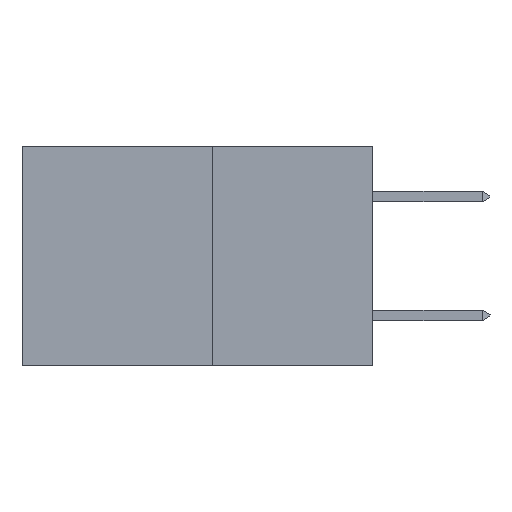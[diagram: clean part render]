
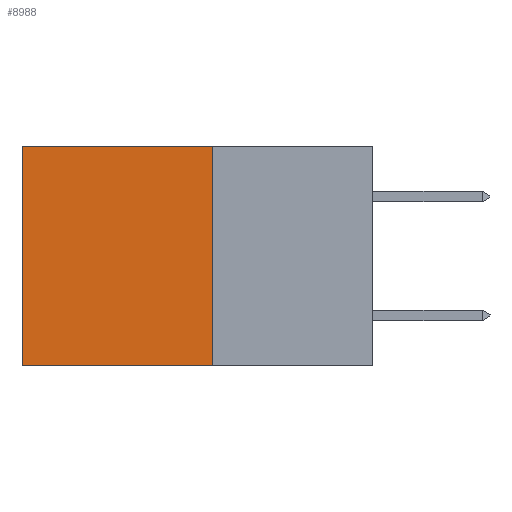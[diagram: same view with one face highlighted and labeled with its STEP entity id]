
A CAD part, left-side view. The second image highlights one B-rep face of the part: STEP entity #8988.
In plain terms, the highlighted planar face has unit normal (-1, 0, 0).
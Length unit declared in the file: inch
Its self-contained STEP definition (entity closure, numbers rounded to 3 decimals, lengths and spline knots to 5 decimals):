
#49 = VECTOR ( 'NONE', #12384, 39.37008 ) ;
#641 = PLANE ( 'NONE',  #1783 ) ;
#1199 = LINE ( 'NONE', #19447, #5732 ) ;
#1234 = ORIENTED_EDGE ( 'NONE', *, *, #15398, .T. ) ;
#1783 = AXIS2_PLACEMENT_3D ( 'NONE', #13892, #2591, #15723 ) ;
#2591 = DIRECTION ( 'NONE',  ( 1., 0., 0. ) ) ;
#3339 = CARTESIAN_POINT ( 'NONE',  ( 0.277, 0.59, 0. ) ) ;
#4191 = CARTESIAN_POINT ( 'NONE',  ( 0.277, 0.59, -0.37 ) ) ;
#5003 = ORIENTED_EDGE ( 'NONE', *, *, #9637, .T. ) ;
#5732 = VECTOR ( 'NONE', #14093, 39.37008 ) ;
#6100 = DIRECTION ( 'NONE',  ( 0., 0., -1. ) ) ;
#6184 = EDGE_LOOP ( 'NONE', ( #1234, #13144, #12387, #5003 ) ) ;
#7509 = CARTESIAN_POINT ( 'NONE',  ( 0.277, 0.27, 0. ) ) ;
#8472 = VERTEX_POINT ( 'NONE', #17714 ) ;
#8706 = VECTOR ( 'NONE', #6100, 39.37008 ) ;
#8988 = ADVANCED_FACE ( 'NONE', ( #19661 ), #641, .F. ) ;
#9637 = EDGE_CURVE ( 'NONE', #10360, #16764, #15700, .T. ) ;
#10173 = LINE ( 'NONE', #10915, #49 ) ;
#10360 = VERTEX_POINT ( 'NONE', #7509 ) ;
#10752 = VECTOR ( 'NONE', #23862, 39.37008 ) ;
#10915 = CARTESIAN_POINT ( 'NONE',  ( 0.277, 0.27, -0.37 ) ) ;
#12384 = DIRECTION ( 'NONE',  ( 0., 1., 0. ) ) ;
#12387 = ORIENTED_EDGE ( 'NONE', *, *, #20684, .F. ) ;
#12895 = CARTESIAN_POINT ( 'NONE',  ( 0.277, 0.27, 0. ) ) ;
#13144 = ORIENTED_EDGE ( 'NONE', *, *, #20227, .F. ) ;
#13892 = CARTESIAN_POINT ( 'NONE',  ( 0.277, 0.27, -0.37 ) ) ;
#14093 = DIRECTION ( 'NONE',  ( 0., 0., -1. ) ) ;
#15398 = EDGE_CURVE ( 'NONE', #16764, #23983, #23343, .T. ) ;
#15700 = LINE ( 'NONE', #12895, #10752 ) ;
#15723 = DIRECTION ( 'NONE',  ( 0., 0., -1. ) ) ;
#16764 = VERTEX_POINT ( 'NONE', #3339 ) ;
#17714 = CARTESIAN_POINT ( 'NONE',  ( 0.277, 0.27, -0.37 ) ) ;
#19447 = CARTESIAN_POINT ( 'NONE',  ( 0.277, 0.27, -0.37 ) ) ;
#19661 = FACE_OUTER_BOUND ( 'NONE', #6184, .T. ) ;
#20227 = EDGE_CURVE ( 'NONE', #8472, #23983, #10173, .T. ) ;
#20684 = EDGE_CURVE ( 'NONE', #10360, #8472, #1199, .T. ) ;
#22438 = CARTESIAN_POINT ( 'NONE',  ( 0.277, 0.59, -0.37 ) ) ;
#23343 = LINE ( 'NONE', #4191, #8706 ) ;
#23862 = DIRECTION ( 'NONE',  ( 0., 1., 0. ) ) ;
#23983 = VERTEX_POINT ( 'NONE', #22438 ) ;
